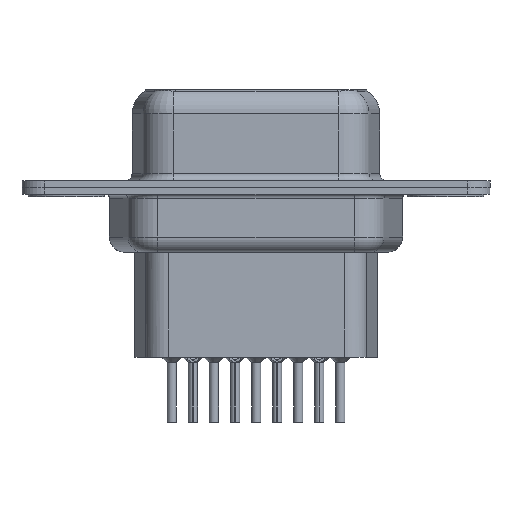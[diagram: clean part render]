
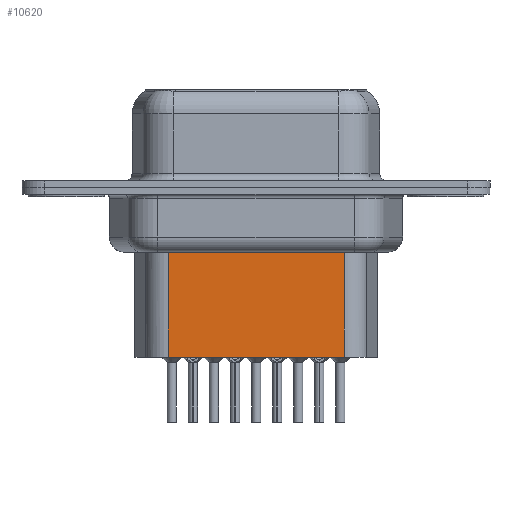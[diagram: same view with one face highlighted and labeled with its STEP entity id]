
A CAD part, front view. The second image highlights one B-rep face of the part: STEP entity #10620.
In plain terms, the highlighted planar face has unit normal (0, -1, 0).
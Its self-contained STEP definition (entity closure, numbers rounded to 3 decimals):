
#906 = EDGE_CURVE ( 'NONE', #13989, #17736, #7733, .T. ) ;
#1647 = DIRECTION ( 'NONE',  ( -1., 0., 0. ) ) ;
#2488 = DIRECTION ( 'NONE',  ( 0., 0., -1. ) ) ;
#2489 = FACE_OUTER_BOUND ( 'NONE', #8328, .T. ) ;
#2715 = EDGE_CURVE ( 'NONE', #12233, #13989, #16202, .T. ) ;
#3243 = VECTOR ( 'NONE', #8696, 1000. ) ;
#3325 = CARTESIAN_POINT ( 'NONE',  ( 6.706, -3.5, -11.15 ) ) ;
#3880 = VECTOR ( 'NONE', #1647, 1000. ) ;
#4045 = ORIENTED_EDGE ( 'NONE', *, *, #2715, .F. ) ;
#4051 = DIRECTION ( 'NONE',  ( -1., 0., 0. ) ) ;
#4342 = CARTESIAN_POINT ( 'NONE',  ( 18.294, -3.5, -11.15 ) ) ;
#5208 = CARTESIAN_POINT ( 'NONE',  ( 6.706, -3.5, -3.1 ) ) ;
#5236 = CARTESIAN_POINT ( 'NONE',  ( 6.706, -3.5, -4.097 ) ) ;
#5361 = CARTESIAN_POINT ( 'NONE',  ( 6.459, -3.5, -4.097 ) ) ;
#5705 = AXIS2_PLACEMENT_3D ( 'NONE', #5208, #19318, #6722 ) ;
#6516 = VECTOR ( 'NONE', #2488, 1000. ) ;
#6722 = DIRECTION ( 'NONE',  ( 1., 0., 0. ) ) ;
#6912 = VERTEX_POINT ( 'NONE', #5236 ) ;
#7267 = VECTOR ( 'NONE', #4051, 1000. ) ;
#7733 = LINE ( 'NONE', #3325, #3880 ) ;
#8317 = CARTESIAN_POINT ( 'NONE',  ( 18.294, -3.5, -3.1 ) ) ;
#8328 = EDGE_LOOP ( 'NONE', ( #4045, #14386, #17651, #13690 ) ) ;
#8696 = DIRECTION ( 'NONE',  ( 0., 0., -1. ) ) ;
#9834 = EDGE_CURVE ( 'NONE', #12233, #6912, #14685, .T. ) ;
#10620 = ADVANCED_FACE ( 'NONE', ( #2489 ), #13215, .T. ) ;
#10856 = EDGE_CURVE ( 'NONE', #6912, #17736, #13612, .T. ) ;
#11208 = CARTESIAN_POINT ( 'NONE',  ( 18.294, -3.5, -4.097 ) ) ;
#12233 = VERTEX_POINT ( 'NONE', #11208 ) ;
#13215 = PLANE ( 'NONE',  #5705 ) ;
#13612 = LINE ( 'NONE', #19511, #3243 ) ;
#13690 = ORIENTED_EDGE ( 'NONE', *, *, #906, .F. ) ;
#13989 = VERTEX_POINT ( 'NONE', #4342 ) ;
#14386 = ORIENTED_EDGE ( 'NONE', *, *, #9834, .T. ) ;
#14685 = LINE ( 'NONE', #5361, #7267 ) ;
#15892 = CARTESIAN_POINT ( 'NONE',  ( 6.706, -3.5, -11.15 ) ) ;
#16202 = LINE ( 'NONE', #8317, #6516 ) ;
#17651 = ORIENTED_EDGE ( 'NONE', *, *, #10856, .T. ) ;
#17736 = VERTEX_POINT ( 'NONE', #15892 ) ;
#19318 = DIRECTION ( 'NONE',  ( 0., -1., 0. ) ) ;
#19511 = CARTESIAN_POINT ( 'NONE',  ( 6.706, -3.5, -3.1 ) ) ;
